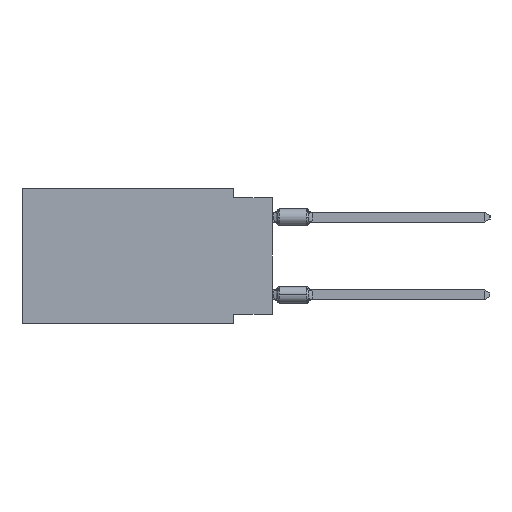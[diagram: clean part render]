
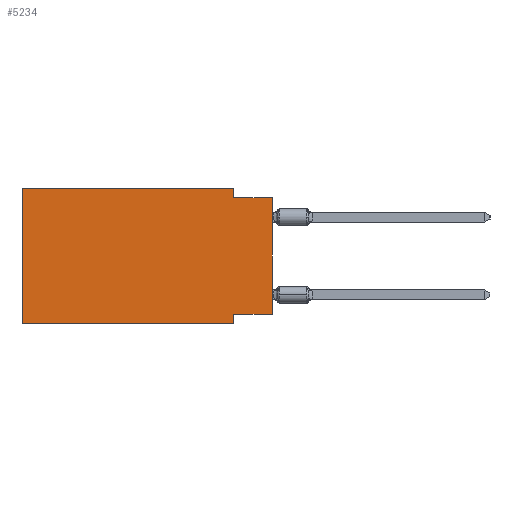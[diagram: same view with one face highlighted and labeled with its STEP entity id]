
A CAD part, left-side view. The second image highlights one B-rep face of the part: STEP entity #5234.
In plain terms, the highlighted planar face has unit normal (-1, 0, 0).
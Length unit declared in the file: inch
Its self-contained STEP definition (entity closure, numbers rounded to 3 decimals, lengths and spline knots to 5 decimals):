
#353 = DIRECTION ( 'NONE',  ( 0., 0., 1. ) ) ;
#377 = LINE ( 'NONE', #45753, #13457 ) ;
#414 = CARTESIAN_POINT ( 'NONE',  ( 0., 0.645, -0.35 ) ) ;
#422 = ORIENTED_EDGE ( 'NONE', *, *, #43603, .F. ) ;
#946 = VECTOR ( 'NONE', #37574, 39.37008 ) ;
#2567 = LINE ( 'NONE', #47156, #27666 ) ;
#3120 = EDGE_CURVE ( 'NONE', #45878, #45267, #377, .T. ) ;
#3576 = VECTOR ( 'NONE', #36420, 39.37008 ) ;
#3936 = CARTESIAN_POINT ( 'NONE',  ( 0., 0., -0.025 ) ) ;
#5234 = ADVANCED_FACE ( 'NONE', ( #16538 ), #41812, .F. ) ;
#5678 = DIRECTION ( 'NONE',  ( 1., 0., 0. ) ) ;
#5766 = VERTEX_POINT ( 'NONE', #18760 ) ;
#6379 = VERTEX_POINT ( 'NONE', #40342 ) ;
#6800 = DIRECTION ( 'NONE',  ( 0., 0., 1. ) ) ;
#7318 = VECTOR ( 'NONE', #6800, 39.37008 ) ;
#8611 = CARTESIAN_POINT ( 'NONE',  ( 0., 0.645, 0. ) ) ;
#8984 = ORIENTED_EDGE ( 'NONE', *, *, #11148, .F. ) ;
#9858 = ORIENTED_EDGE ( 'NONE', *, *, #3120, .F. ) ;
#10341 = CARTESIAN_POINT ( 'NONE',  ( 0., 0.1, -0.35 ) ) ;
#10383 = ORIENTED_EDGE ( 'NONE', *, *, #49249, .T. ) ;
#11011 = CARTESIAN_POINT ( 'NONE',  ( 0., 0., 0. ) ) ;
#11148 = EDGE_CURVE ( 'NONE', #45267, #6379, #34441, .T. ) ;
#11647 = EDGE_LOOP ( 'NONE', ( #35873, #36748, #8984, #9858, #24710, #10383, #422, #31664 ) ) ;
#11718 = CARTESIAN_POINT ( 'NONE',  ( 0., 0.1, -0.325 ) ) ;
#13457 = VECTOR ( 'NONE', #29108, 39.37008 ) ;
#14710 = LINE ( 'NONE', #11011, #7318 ) ;
#16136 = CARTESIAN_POINT ( 'NONE',  ( 0., 0., -0.325 ) ) ;
#16538 = FACE_OUTER_BOUND ( 'NONE', #11647, .T. ) ;
#17272 = LINE ( 'NONE', #33417, #43367 ) ;
#18760 = CARTESIAN_POINT ( 'NONE',  ( 0., 0.1, -0.35 ) ) ;
#19317 = VERTEX_POINT ( 'NONE', #3936 ) ;
#19464 = EDGE_CURVE ( 'NONE', #6379, #19317, #24235, .T. ) ;
#19920 = VECTOR ( 'NONE', #50546, 39.37008 ) ;
#20750 = DIRECTION ( 'NONE',  ( 0., 0., -1. ) ) ;
#20850 = DIRECTION ( 'NONE',  ( 0., 1., 0. ) ) ;
#21402 = VERTEX_POINT ( 'NONE', #47364 ) ;
#24235 = LINE ( 'NONE', #44570, #3576 ) ;
#24710 = ORIENTED_EDGE ( 'NONE', *, *, #38489, .F. ) ;
#26744 = CARTESIAN_POINT ( 'NONE',  ( 0., 0.1, 0. ) ) ;
#27666 = VECTOR ( 'NONE', #353, 39.37008 ) ;
#28315 = VERTEX_POINT ( 'NONE', #11718 ) ;
#29108 = DIRECTION ( 'NONE',  ( 0., -1., 0. ) ) ;
#29440 = DIRECTION ( 'NONE',  ( 0., -1., 0. ) ) ;
#30136 = LINE ( 'NONE', #10341, #946 ) ;
#31664 = ORIENTED_EDGE ( 'NONE', *, *, #39719, .F. ) ;
#32685 = CARTESIAN_POINT ( 'NONE',  ( 0., 0.645, 0. ) ) ;
#33417 = CARTESIAN_POINT ( 'NONE',  ( 0., 0.645, -0.35 ) ) ;
#33970 = LINE ( 'NONE', #16136, #41241 ) ;
#34065 = CARTESIAN_POINT ( 'NONE',  ( 0., 0.1, 0. ) ) ;
#34441 = LINE ( 'NONE', #26744, #19920 ) ;
#35873 = ORIENTED_EDGE ( 'NONE', *, *, #51418, .T. ) ;
#36420 = DIRECTION ( 'NONE',  ( 0., -1., 0. ) ) ;
#36748 = ORIENTED_EDGE ( 'NONE', *, *, #19464, .F. ) ;
#37574 = DIRECTION ( 'NONE',  ( 0., 0., -1. ) ) ;
#38489 = EDGE_CURVE ( 'NONE', #42312, #45878, #2567, .T. ) ;
#39719 = EDGE_CURVE ( 'NONE', #21402, #28315, #33970, .T. ) ;
#40342 = CARTESIAN_POINT ( 'NONE',  ( 0., 0.1, -0.025 ) ) ;
#41241 = VECTOR ( 'NONE', #20850, 39.37008 ) ;
#41812 = PLANE ( 'NONE',  #49785 ) ;
#42312 = VERTEX_POINT ( 'NONE', #414 ) ;
#43367 = VECTOR ( 'NONE', #29440, 39.37008 ) ;
#43603 = EDGE_CURVE ( 'NONE', #28315, #5766, #30136, .T. ) ;
#44570 = CARTESIAN_POINT ( 'NONE',  ( 0., 0., -0.025 ) ) ;
#45267 = VERTEX_POINT ( 'NONE', #34065 ) ;
#45753 = CARTESIAN_POINT ( 'NONE',  ( 0., 0.645, 0. ) ) ;
#45878 = VERTEX_POINT ( 'NONE', #8611 ) ;
#47156 = CARTESIAN_POINT ( 'NONE',  ( 0., 0.645, 0. ) ) ;
#47364 = CARTESIAN_POINT ( 'NONE',  ( 0., 0., -0.325 ) ) ;
#49249 = EDGE_CURVE ( 'NONE', #42312, #5766, #17272, .T. ) ;
#49785 = AXIS2_PLACEMENT_3D ( 'NONE', #32685, #5678, #20750 ) ;
#50546 = DIRECTION ( 'NONE',  ( 0., 0., -1. ) ) ;
#51418 = EDGE_CURVE ( 'NONE', #21402, #19317, #14710, .T. ) ;
